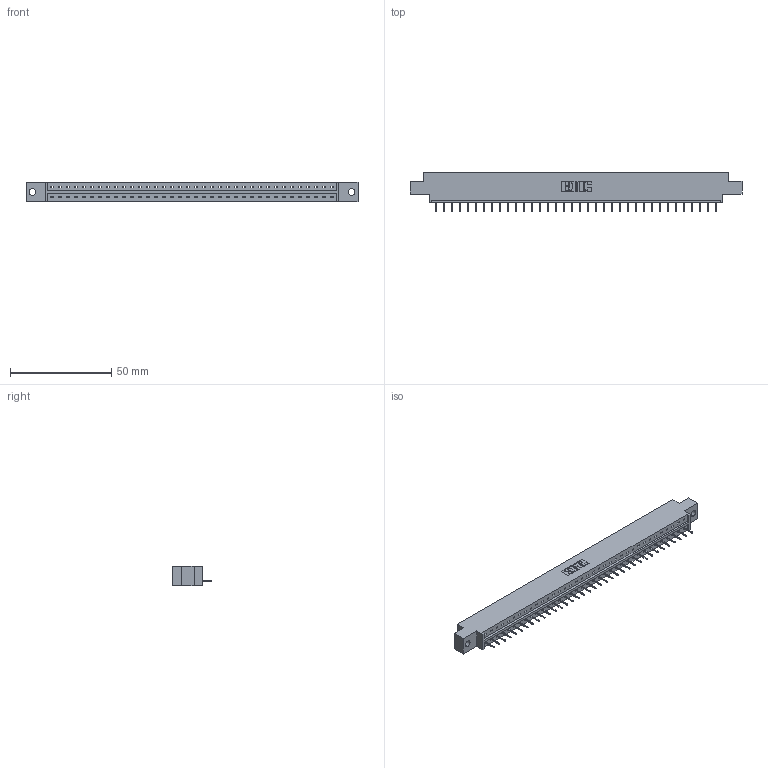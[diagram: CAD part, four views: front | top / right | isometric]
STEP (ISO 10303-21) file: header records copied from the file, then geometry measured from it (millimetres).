
FILE_DESCRIPTION (( 'STEP AP203' ), '1' );
FILE_NAME ('333-036-524-602.STEP', '2018-08-03T00:46:01', ( '' ), ( '' ), 'SwSTEP 2.0', 'SolidWorks 2016', '' );
FILE_SCHEMA (( 'CONFIG_CONTROL_DESIGN' ));
Length unit declared in the file: inch
Products named in the file (3): 333 Part_Offset - .128 Dia; 345-292-001_345-293-124; 333-036-524-602
Assembly tree (37 placements, depth 2):
  333-036-524-602
    333 Part_Offset - .128 Dia
    345-292-001_345-293-124  x36
Bounding box: 164.19 x 19.69 x 9.4 mm (x, y, z)
Volume: 16063.4 mm3; surface area: 16778.1 mm2
Topology: 37 solids, 37 shells, 2350 faces, 6803 edges, 4390 vertices
Faces by surface type: plane 1802, cylinder 548
Entity records: 22993 total; most frequent: CARTESIAN_POINT 3974, ORIENTED_EDGE 3946, DIRECTION 3365, EDGE_CURVE 1973, LINE 1849, VECTOR 1849, VERTEX_POINT 1310, AXIS2_PLACEMENT_3D 758
